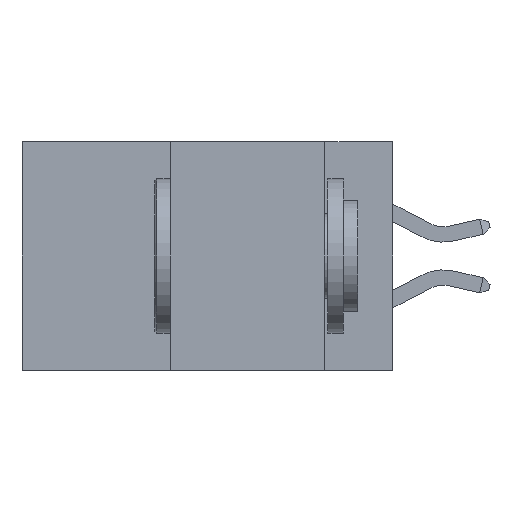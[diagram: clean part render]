
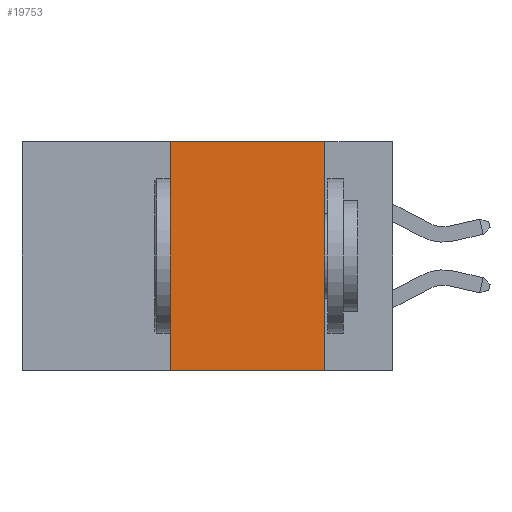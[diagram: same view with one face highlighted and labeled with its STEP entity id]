
A CAD part, left-side view. The second image highlights one B-rep face of the part: STEP entity #19753.
In plain terms, the highlighted planar face has unit normal (-1, 0, 0).
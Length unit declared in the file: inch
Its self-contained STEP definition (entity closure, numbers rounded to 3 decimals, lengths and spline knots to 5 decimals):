
#23 = CARTESIAN_POINT ( 'NONE',  ( 0., 0.6, -0.37 ) ) ;
#172 = EDGE_CURVE ( 'NONE', #17731, #4761, #20465, .T. ) ;
#482 = CARTESIAN_POINT ( 'NONE',  ( 0., 0.36, 0. ) ) ;
#1232 = CARTESIAN_POINT ( 'NONE',  ( 0., 0.6, 0. ) ) ;
#2705 = DIRECTION ( 'NONE',  ( 0., -1., 0. ) ) ;
#2765 = CARTESIAN_POINT ( 'NONE',  ( 0., 0.11, 0. ) ) ;
#2919 = DIRECTION ( 'NONE',  ( 1., 0., 0. ) ) ;
#4561 = DIRECTION ( 'NONE',  ( 0., 0., -1. ) ) ;
#4761 = VERTEX_POINT ( 'NONE', #12099 ) ;
#4829 = VERTEX_POINT ( 'NONE', #10428 ) ;
#7025 = VERTEX_POINT ( 'NONE', #482 ) ;
#8665 = EDGE_LOOP ( 'NONE', ( #11290, #11791, #20745, #12867 ) ) ;
#8667 = VECTOR ( 'NONE', #4561, 39.37008 ) ;
#8802 = VECTOR ( 'NONE', #13395, 39.37008 ) ;
#9184 = EDGE_CURVE ( 'NONE', #4829, #4761, #12062, .T. ) ;
#9433 = CARTESIAN_POINT ( 'NONE',  ( 0., 0.36, 0. ) ) ;
#9493 = AXIS2_PLACEMENT_3D ( 'NONE', #18201, #2919, #14908 ) ;
#10428 = CARTESIAN_POINT ( 'NONE',  ( 0., 0.11, 0. ) ) ;
#11290 = ORIENTED_EDGE ( 'NONE', *, *, #9184, .F. ) ;
#11791 = ORIENTED_EDGE ( 'NONE', *, *, #19157, .F. ) ;
#12062 = LINE ( 'NONE', #2765, #8667 ) ;
#12099 = CARTESIAN_POINT ( 'NONE',  ( 0., 0.11, -0.37 ) ) ;
#12867 = ORIENTED_EDGE ( 'NONE', *, *, #172, .T. ) ;
#13030 = VECTOR ( 'NONE', #14511, 39.37008 ) ;
#13395 = DIRECTION ( 'NONE',  ( 0., -1., 0. ) ) ;
#14355 = FACE_OUTER_BOUND ( 'NONE', #8665, .T. ) ;
#14511 = DIRECTION ( 'NONE',  ( 0., 0., 1. ) ) ;
#14908 = DIRECTION ( 'NONE',  ( 0., 0., -1. ) ) ;
#15996 = VECTOR ( 'NONE', #2705, 39.37008 ) ;
#17216 = LINE ( 'NONE', #1232, #8802 ) ;
#17731 = VERTEX_POINT ( 'NONE', #21317 ) ;
#18201 = CARTESIAN_POINT ( 'NONE',  ( 0., 0.6, 0. ) ) ;
#18917 = EDGE_CURVE ( 'NONE', #17731, #7025, #21451, .T. ) ;
#19157 = EDGE_CURVE ( 'NONE', #7025, #4829, #17216, .T. ) ;
#19753 = ADVANCED_FACE ( 'NONE', ( #14355 ), #19911, .F. ) ;
#19911 = PLANE ( 'NONE',  #9493 ) ;
#20465 = LINE ( 'NONE', #23, #15996 ) ;
#20745 = ORIENTED_EDGE ( 'NONE', *, *, #18917, .F. ) ;
#21317 = CARTESIAN_POINT ( 'NONE',  ( 0., 0.36, -0.37 ) ) ;
#21451 = LINE ( 'NONE', #9433, #13030 ) ;
